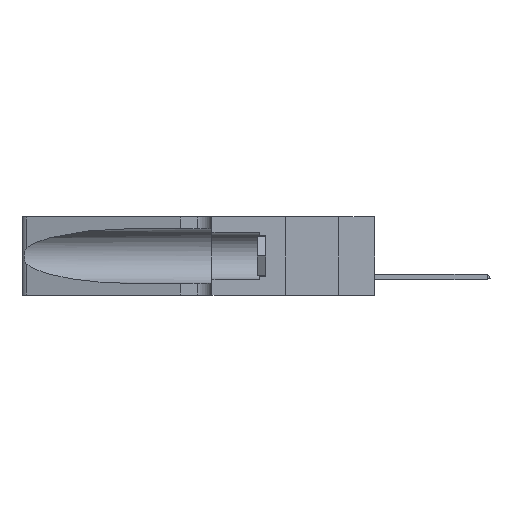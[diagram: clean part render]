
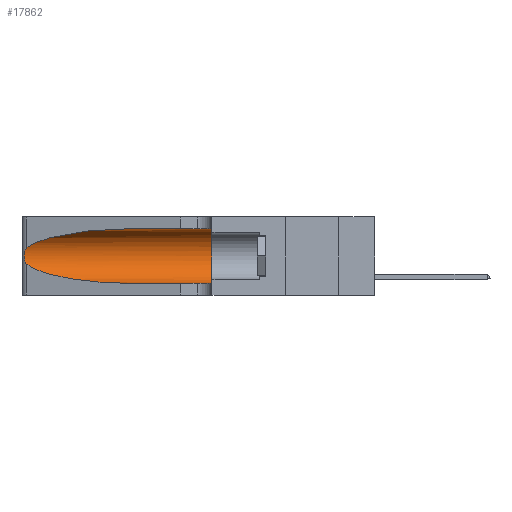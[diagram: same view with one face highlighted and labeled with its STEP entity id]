
A CAD part, left-side view. The second image highlights one B-rep face of the part: STEP entity #17862.
In plain terms, the highlighted cylindrical face has radius 3.308 mm (diameter 6.617 mm), a partial arc.
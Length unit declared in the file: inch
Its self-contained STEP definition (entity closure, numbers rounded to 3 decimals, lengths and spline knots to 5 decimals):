
#372 = VECTOR ( 'NONE', #15413, 39.37008 ) ;
#926 = CARTESIAN_POINT ( 'NONE',  ( 0.2373, 1.15595, 0.08982 ) ) ;
#1258 = VERTEX_POINT ( 'NONE', #32188 ) ;
#3328 = CARTESIAN_POINT ( 'NONE',  ( 0.1305, 1.61858, 0.05475 ) ) ;
#3939 = EDGE_CURVE ( 'NONE', #20397, #17307, #13222, .T. ) ;
#3987 = FACE_OUTER_BOUND ( 'NONE', #30725, .T. ) ;
#5077 = CARTESIAN_POINT ( 'NONE',  ( 0.18966, 0.96281, 0.05475 ) ) ;
#5142 = CARTESIAN_POINT ( 'NONE',  ( 0.25487, 1.22718, 0.22369 ) ) ;
#7000 = ORIENTED_EDGE ( 'NONE', *, *, #14052, .T. ) ;
#9554 =( BOUNDED_CURVE ( )  B_SPLINE_CURVE ( 3, ( #51031, #16218, #31879, #12888 ),
 .UNSPECIFIED., .F., .T. ) 
 B_SPLINE_CURVE_WITH_KNOTS ( ( 4, 4 ),
 ( 1.5708, 2.84003 ),
 .UNSPECIFIED. ) 
 CURVE ( )  GEOMETRIC_REPRESENTATION_ITEM ( )  RATIONAL_B_SPLINE_CURVE ( ( 1., 0.87, 0.87, 1. ) ) 
 REPRESENTATION_ITEM ( '' )  );
#11532 = CARTESIAN_POINT ( 'NONE',  ( 0.1305, 1.61858, 0.31525 ) ) ;
#12888 = CARTESIAN_POINT ( 'NONE',  ( 0.25487, 1.22718, 0.22369 ) ) ;
#13222 = CIRCLE ( 'NONE', #47488, 0.13025 ) ;
#14052 = EDGE_CURVE ( 'NONE', #18223, #20759, #42555, .T. ) ;
#14498 = CARTESIAN_POINT ( 'NONE',  ( 0.25487, 1.22718, 0.14631 ) ) ;
#15413 = DIRECTION ( 'NONE',  ( 0., -1., 0. ) ) ;
#15552 = CARTESIAN_POINT ( 'NONE',  ( 0.1305, 1.61858, 0.185 ) ) ;
#16218 = CARTESIAN_POINT ( 'NONE',  ( 0.18966, 0.96281, 0.31525 ) ) ;
#17037 = CARTESIAN_POINT ( 'NONE',  ( 0.25787, 1.23484, 0.2124 ) ) ;
#17307 = VERTEX_POINT ( 'NONE', #48441 ) ;
#17377 = CARTESIAN_POINT ( 'NONE',  ( 0.25856, 1.23593, 0.16098 ) ) ;
#17862 = ADVANCED_FACE ( 'NONE', ( #3987 ), #49757, .F. ) ;
#18223 = VERTEX_POINT ( 'NONE', #50577 ) ;
#19848 = EDGE_CURVE ( 'NONE', #20759, #23579, #47899, .T. ) ;
#20397 = VERTEX_POINT ( 'NONE', #33920 ) ;
#20436 = AXIS2_PLACEMENT_3D ( 'NONE', #15552, #51176, #27381 ) ;
#20759 = VERTEX_POINT ( 'NONE', #41089 ) ;
#20973 = CARTESIAN_POINT ( 'NONE',  ( 0.25854, 1.2359, 0.20912 ) ) ;
#21768 = LINE ( 'NONE', #11532, #42867 ) ;
#23579 = VERTEX_POINT ( 'NONE', #43846 ) ;
#24942 = CARTESIAN_POINT ( 'NONE',  ( 0.26018, 1.23835, 0.19895 ) ) ;
#25470 = CARTESIAN_POINT ( 'NONE',  ( 0.25639, 1.23184, 0.21858 ) ) ;
#25677 = DIRECTION ( 'NONE',  ( 0., 0., 1. ) ) ;
#26346 = CARTESIAN_POINT ( 'NONE',  ( 0.26075, 1.23896, 0.178 ) ) ;
#26525 = EDGE_CURVE ( 'NONE', #1258, #18223, #9554, .T. ) ;
#27381 = DIRECTION ( 'NONE',  ( 0., 0., -1. ) ) ;
#30725 = EDGE_LOOP ( 'NONE', ( #37057, #7000, #42523, #35973, #34889, #36948 ) ) ;
#30751 = CARTESIAN_POINT ( 'NONE',  ( 0.1305, 0.72297, 0.05475 ) ) ;
#31879 = CARTESIAN_POINT ( 'NONE',  ( 0.2373, 1.15595, 0.28018 ) ) ;
#32188 = CARTESIAN_POINT ( 'NONE',  ( 0.1305, 0.72297, 0.31525 ) ) ;
#32305 = CARTESIAN_POINT ( 'NONE',  ( 0.25487, 1.22718, 0.14631 ) ) ;
#33563 = EDGE_CURVE ( 'NONE', #1258, #20397, #21768, .T. ) ;
#33920 = CARTESIAN_POINT ( 'NONE',  ( 0.1305, 0.35, 0.31525 ) ) ;
#34889 = ORIENTED_EDGE ( 'NONE', *, *, #3939, .F. ) ;
#35701 = CARTESIAN_POINT ( 'NONE',  ( 0.25789, 1.23486, 0.15765 ) ) ;
#35973 = ORIENTED_EDGE ( 'NONE', *, *, #50543, .T. ) ;
#36948 = ORIENTED_EDGE ( 'NONE', *, *, #33563, .F. ) ;
#37054 = CARTESIAN_POINT ( 'NONE',  ( 0.1305, 0.35, 0.185 ) ) ;
#37057 = ORIENTED_EDGE ( 'NONE', *, *, #26525, .T. ) ;
#37376 = LINE ( 'NONE', #3328, #372 ) ;
#38832 = CARTESIAN_POINT ( 'NONE',  ( 0.25639, 1.23186, 0.15144 ) ) ;
#40684 = CARTESIAN_POINT ( 'NONE',  ( 0.25555, 1.22994, 0.2215 ) ) ;
#41089 = CARTESIAN_POINT ( 'NONE',  ( 0.25487, 1.22718, 0.14631 ) ) ;
#42523 = ORIENTED_EDGE ( 'NONE', *, *, #19848, .T. ) ;
#42555 = B_SPLINE_CURVE_WITH_KNOTS ( 'NONE', 3,
 ( #5142, #40684, #25470, #17037, #20973, #24942, #46089, #26346, #49504, #17377, #35701, #38832, #50131, #14498 ),
 .UNSPECIFIED., .F., .F.,
 ( 4, 2, 2, 2, 2, 2, 4 ),
 ( 0., 0.00027, 0.00053, 0.00107, 0.0016, 0.00187, 0.00214 ),
 .UNSPECIFIED. ) ;
#42816 = DIRECTION ( 'NONE',  ( 0., -1., 0. ) ) ;
#42867 = VECTOR ( 'NONE', #42816, 39.37008 ) ;
#43846 = CARTESIAN_POINT ( 'NONE',  ( 0.1305, 0.72297, 0.05475 ) ) ;
#45037 = DIRECTION ( 'NONE',  ( 0., 1., 0. ) ) ;
#46089 = CARTESIAN_POINT ( 'NONE',  ( 0.26075, 1.23896, 0.19203 ) ) ;
#47488 = AXIS2_PLACEMENT_3D ( 'NONE', #37054, #45037, #25677 ) ;
#47899 =( BOUNDED_CURVE ( )  B_SPLINE_CURVE ( 3, ( #32305, #926, #5077, #30751 ),
 .UNSPECIFIED., .F., .F. ) 
 B_SPLINE_CURVE_WITH_KNOTS ( ( 4, 4 ),
 ( 3.44316, 4.71239 ),
 .UNSPECIFIED. ) 
 CURVE ( )  GEOMETRIC_REPRESENTATION_ITEM ( )  RATIONAL_B_SPLINE_CURVE ( ( 1., 0.87, 0.87, 1. ) ) 
 REPRESENTATION_ITEM ( '' )  );
#48441 = CARTESIAN_POINT ( 'NONE',  ( 0.1305, 0.35, 0.05475 ) ) ;
#49504 = CARTESIAN_POINT ( 'NONE',  ( 0.26017, 1.23833, 0.17102 ) ) ;
#49757 = CYLINDRICAL_SURFACE ( 'NONE', #20436, 0.13025 ) ;
#50131 = CARTESIAN_POINT ( 'NONE',  ( 0.25555, 1.22993, 0.14849 ) ) ;
#50543 = EDGE_CURVE ( 'NONE', #23579, #17307, #37376, .T. ) ;
#50577 = CARTESIAN_POINT ( 'NONE',  ( 0.25487, 1.22718, 0.22369 ) ) ;
#51031 = CARTESIAN_POINT ( 'NONE',  ( 0.1305, 0.72297, 0.31525 ) ) ;
#51176 = DIRECTION ( 'NONE',  ( 0., -1., 0. ) ) ;
